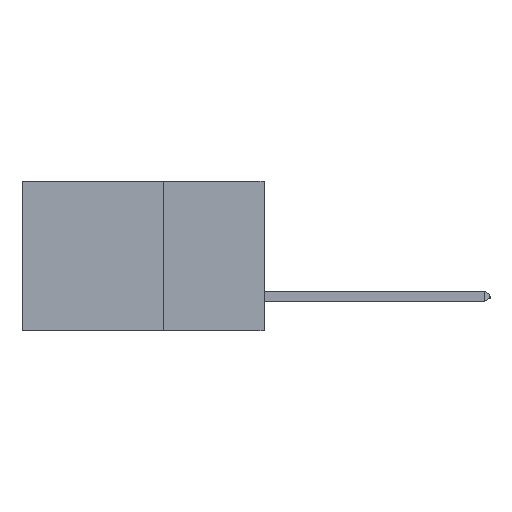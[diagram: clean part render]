
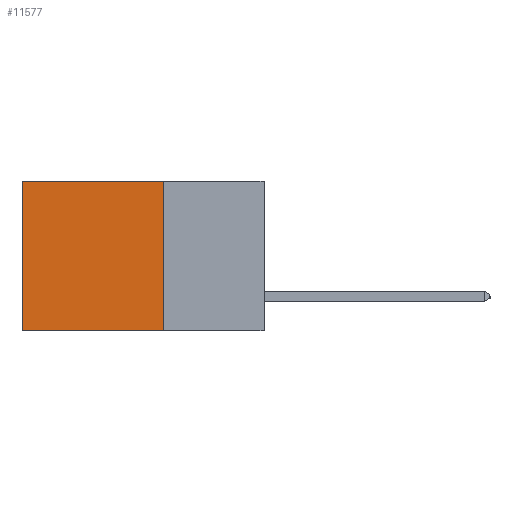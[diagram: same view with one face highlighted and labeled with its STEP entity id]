
A CAD part, left-side view. The second image highlights one B-rep face of the part: STEP entity #11577.
In plain terms, the highlighted planar face has unit normal (-1, 0, 0).
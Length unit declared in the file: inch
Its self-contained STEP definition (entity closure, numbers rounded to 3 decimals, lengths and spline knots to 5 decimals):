
#8 = EDGE_CURVE ( 'NONE', #2536, #19090, #18206, .T. ) ;
#832 = CARTESIAN_POINT ( 'NONE',  ( 0.298, 0.6, -0.37 ) ) ;
#1127 = FACE_OUTER_BOUND ( 'NONE', #3894, .T. ) ;
#1213 = VECTOR ( 'NONE', #17416, 39.37008 ) ;
#1672 = PLANE ( 'NONE',  #10150 ) ;
#2536 = VERTEX_POINT ( 'NONE', #3399 ) ;
#3399 = CARTESIAN_POINT ( 'NONE',  ( 0.298, 0.25, 0. ) ) ;
#3894 = EDGE_LOOP ( 'NONE', ( #16097, #15769, #10225, #6547 ) ) ;
#4018 = CARTESIAN_POINT ( 'NONE',  ( 0.298, 0.6, 0. ) ) ;
#4306 = CARTESIAN_POINT ( 'NONE',  ( 0.298, 0.6, 0. ) ) ;
#4680 = LINE ( 'NONE', #19169, #8626 ) ;
#5375 = CARTESIAN_POINT ( 'NONE',  ( 0.298, 0.25, 0. ) ) ;
#6547 = ORIENTED_EDGE ( 'NONE', *, *, #20865, .T. ) ;
#7027 = VECTOR ( 'NONE', #16817, 39.37008 ) ;
#8377 = DIRECTION ( 'NONE',  ( 1., 0., 0. ) ) ;
#8626 = VECTOR ( 'NONE', #12667, 39.37008 ) ;
#8790 = VERTEX_POINT ( 'NONE', #832 ) ;
#9398 = VERTEX_POINT ( 'NONE', #4018 ) ;
#9469 = CARTESIAN_POINT ( 'NONE',  ( 0.298, 0.25, -0.37 ) ) ;
#10063 = EDGE_CURVE ( 'NONE', #9398, #8790, #18709, .T. ) ;
#10150 = AXIS2_PLACEMENT_3D ( 'NONE', #18102, #8377, #19784 ) ;
#10225 = ORIENTED_EDGE ( 'NONE', *, *, #8, .F. ) ;
#11175 = DIRECTION ( 'NONE',  ( 0., 0., -1. ) ) ;
#11577 = ADVANCED_FACE ( 'NONE', ( #1127 ), #1672, .F. ) ;
#12667 = DIRECTION ( 'NONE',  ( 0., 1., 0. ) ) ;
#13249 = EDGE_CURVE ( 'NONE', #19090, #8790, #4680, .T. ) ;
#13884 = VECTOR ( 'NONE', #11175, 39.37008 ) ;
#14001 = CARTESIAN_POINT ( 'NONE',  ( 0.298, 0.25, 0. ) ) ;
#15769 = ORIENTED_EDGE ( 'NONE', *, *, #13249, .F. ) ;
#16097 = ORIENTED_EDGE ( 'NONE', *, *, #10063, .T. ) ;
#16191 = LINE ( 'NONE', #5375, #7027 ) ;
#16817 = DIRECTION ( 'NONE',  ( 0., 1., 0. ) ) ;
#17416 = DIRECTION ( 'NONE',  ( 0., 0., -1. ) ) ;
#18102 = CARTESIAN_POINT ( 'NONE',  ( 0.298, 0.25, 0. ) ) ;
#18206 = LINE ( 'NONE', #14001, #13884 ) ;
#18709 = LINE ( 'NONE', #4306, #1213 ) ;
#19090 = VERTEX_POINT ( 'NONE', #9469 ) ;
#19169 = CARTESIAN_POINT ( 'NONE',  ( 0.298, 0.25, -0.37 ) ) ;
#19784 = DIRECTION ( 'NONE',  ( 0., 0., -1. ) ) ;
#20865 = EDGE_CURVE ( 'NONE', #2536, #9398, #16191, .T. ) ;
